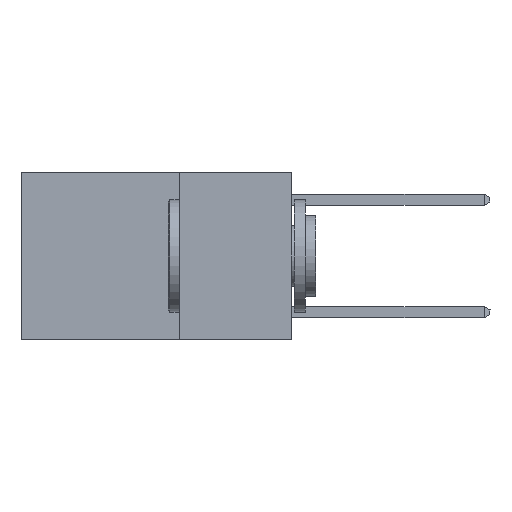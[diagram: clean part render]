
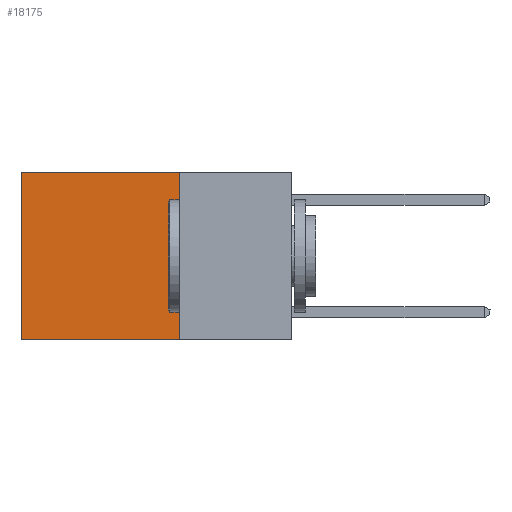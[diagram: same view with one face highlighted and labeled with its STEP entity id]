
A CAD part, left-side view. The second image highlights one B-rep face of the part: STEP entity #18175.
In plain terms, the highlighted planar face has unit normal (-1, 0, 0).
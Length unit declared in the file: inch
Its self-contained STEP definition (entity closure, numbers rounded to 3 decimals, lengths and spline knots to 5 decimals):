
#1487 = DIRECTION ( 'NONE',  ( 0., 0., -1. ) ) ;
#2210 = CARTESIAN_POINT ( 'NONE',  ( 0.2625, 0.25, 0. ) ) ;
#3915 = LINE ( 'NONE', #6577, #27925 ) ;
#4587 = EDGE_CURVE ( 'NONE', #5998, #6724, #15340, .T. ) ;
#4765 = VECTOR ( 'NONE', #17816, 39.37008 ) ;
#5998 = VERTEX_POINT ( 'NONE', #19362 ) ;
#6520 = VERTEX_POINT ( 'NONE', #27315 ) ;
#6577 = CARTESIAN_POINT ( 'NONE',  ( 0.2625, 0.25, -0.37 ) ) ;
#6699 = PLANE ( 'NONE',  #24362 ) ;
#6724 = VERTEX_POINT ( 'NONE', #21096 ) ;
#7492 = ORIENTED_EDGE ( 'NONE', *, *, #21268, .T. ) ;
#7611 = FACE_OUTER_BOUND ( 'NONE', #24827, .T. ) ;
#8289 = ORIENTED_EDGE ( 'NONE', *, *, #15620, .F. ) ;
#8950 = ORIENTED_EDGE ( 'NONE', *, *, #17677, .F. ) ;
#8975 = DIRECTION ( 'NONE',  ( 1., 0., 0. ) ) ;
#9036 = ORIENTED_EDGE ( 'NONE', *, *, #4587, .T. ) ;
#12853 = LINE ( 'NONE', #13283, #4765 ) ;
#13283 = CARTESIAN_POINT ( 'NONE',  ( 0.2625, 0.25, 0. ) ) ;
#13539 = CARTESIAN_POINT ( 'NONE',  ( 0.2625, 0.25, 0. ) ) ;
#15340 = LINE ( 'NONE', #13539, #26827 ) ;
#15620 = EDGE_CURVE ( 'NONE', #6520, #22923, #3915, .T. ) ;
#15805 = DIRECTION ( 'NONE',  ( 0., 1., 0. ) ) ;
#17677 = EDGE_CURVE ( 'NONE', #5998, #6520, #12853, .T. ) ;
#17816 = DIRECTION ( 'NONE',  ( 0., 0., -1. ) ) ;
#18175 = ADVANCED_FACE ( 'NONE', ( #7611 ), #6699, .F. ) ;
#19362 = CARTESIAN_POINT ( 'NONE',  ( 0.2625, 0.25, 0. ) ) ;
#21096 = CARTESIAN_POINT ( 'NONE',  ( 0.2625, 0.6, 0. ) ) ;
#21268 = EDGE_CURVE ( 'NONE', #6724, #22923, #28836, .T. ) ;
#22222 = VECTOR ( 'NONE', #1487, 39.37008 ) ;
#22434 = DIRECTION ( 'NONE',  ( 0., 1., 0. ) ) ;
#22923 = VERTEX_POINT ( 'NONE', #24692 ) ;
#24043 = CARTESIAN_POINT ( 'NONE',  ( 0.2625, 0.6, 0. ) ) ;
#24362 = AXIS2_PLACEMENT_3D ( 'NONE', #2210, #8975, #24856 ) ;
#24692 = CARTESIAN_POINT ( 'NONE',  ( 0.2625, 0.6, -0.37 ) ) ;
#24827 = EDGE_LOOP ( 'NONE', ( #7492, #8289, #8950, #9036 ) ) ;
#24856 = DIRECTION ( 'NONE',  ( 0., 0., -1. ) ) ;
#26827 = VECTOR ( 'NONE', #15805, 39.37008 ) ;
#27315 = CARTESIAN_POINT ( 'NONE',  ( 0.2625, 0.25, -0.37 ) ) ;
#27925 = VECTOR ( 'NONE', #22434, 39.37008 ) ;
#28836 = LINE ( 'NONE', #24043, #22222 ) ;
